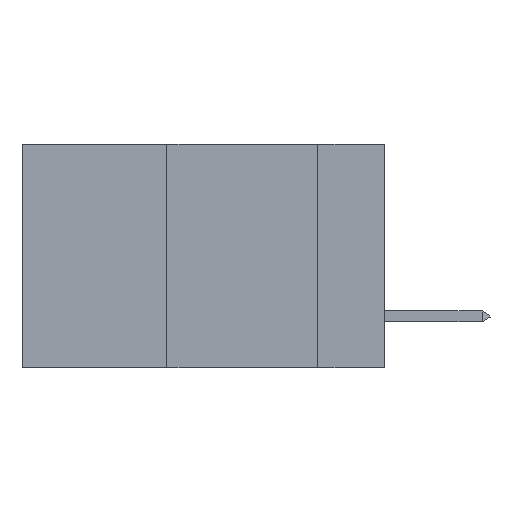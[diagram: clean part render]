
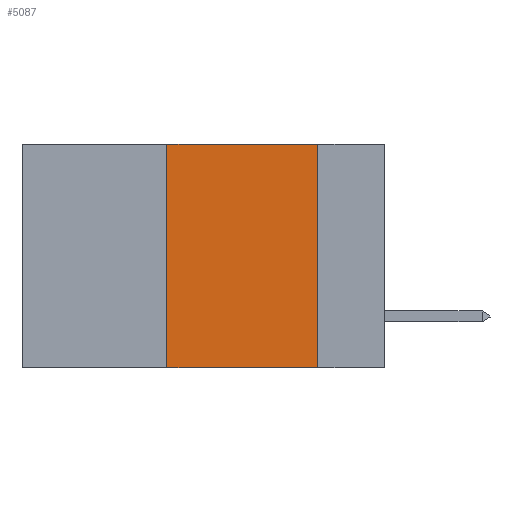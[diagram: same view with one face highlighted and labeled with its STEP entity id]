
A CAD part, left-side view. The second image highlights one B-rep face of the part: STEP entity #5087.
In plain terms, the highlighted planar face has unit normal (-1, 0, 0).
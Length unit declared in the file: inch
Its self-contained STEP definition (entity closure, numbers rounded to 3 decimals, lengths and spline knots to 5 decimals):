
#1336 = ORIENTED_EDGE ( 'NONE', *, *, #5442, .F. ) ;
#1429 = CARTESIAN_POINT ( 'NONE',  ( 0., 0.6, -0.37 ) ) ;
#1559 = LINE ( 'NONE', #3818, #13068 ) ;
#1743 = DIRECTION ( 'NONE',  ( 0., 0., 1. ) ) ;
#3305 = DIRECTION ( 'NONE',  ( 0., -1., 0. ) ) ;
#3705 = FACE_OUTER_BOUND ( 'NONE', #15469, .T. ) ;
#3818 = CARTESIAN_POINT ( 'NONE',  ( 0., 0.11, 0. ) ) ;
#4526 = CARTESIAN_POINT ( 'NONE',  ( 0., 0.6, 0. ) ) ;
#4666 = LINE ( 'NONE', #4526, #16384 ) ;
#4720 = VERTEX_POINT ( 'NONE', #7109 ) ;
#4814 = CARTESIAN_POINT ( 'NONE',  ( 0., 0.6, 0. ) ) ;
#5087 = ADVANCED_FACE ( 'NONE', ( #3705 ), #9902, .F. ) ;
#5442 = EDGE_CURVE ( 'NONE', #5704, #4720, #1559, .T. ) ;
#5704 = VERTEX_POINT ( 'NONE', #6829 ) ;
#6124 = DIRECTION ( 'NONE',  ( 1., 0., 0. ) ) ;
#6217 = CARTESIAN_POINT ( 'NONE',  ( 0., 0.36, 0. ) ) ;
#6248 = EDGE_CURVE ( 'NONE', #13581, #12804, #13221, .T. ) ;
#6829 = CARTESIAN_POINT ( 'NONE',  ( 0., 0.11, 0. ) ) ;
#6848 = ORIENTED_EDGE ( 'NONE', *, *, #14218, .F. ) ;
#7109 = CARTESIAN_POINT ( 'NONE',  ( 0., 0.11, -0.37 ) ) ;
#7263 = VECTOR ( 'NONE', #1743, 39.37008 ) ;
#7389 = EDGE_CURVE ( 'NONE', #13581, #4720, #12853, .T. ) ;
#8726 = ORIENTED_EDGE ( 'NONE', *, *, #6248, .F. ) ;
#8911 = ORIENTED_EDGE ( 'NONE', *, *, #7389, .T. ) ;
#9166 = DIRECTION ( 'NONE',  ( 0., -1., 0. ) ) ;
#9665 = VECTOR ( 'NONE', #9166, 39.37008 ) ;
#9902 = PLANE ( 'NONE',  #15212 ) ;
#12204 = CARTESIAN_POINT ( 'NONE',  ( 0., 0.36, -0.37 ) ) ;
#12804 = VERTEX_POINT ( 'NONE', #6217 ) ;
#12853 = LINE ( 'NONE', #1429, #9665 ) ;
#13068 = VECTOR ( 'NONE', #16360, 39.37008 ) ;
#13221 = LINE ( 'NONE', #15648, #7263 ) ;
#13581 = VERTEX_POINT ( 'NONE', #12204 ) ;
#14218 = EDGE_CURVE ( 'NONE', #12804, #5704, #4666, .T. ) ;
#14969 = DIRECTION ( 'NONE',  ( 0., 0., -1. ) ) ;
#15212 = AXIS2_PLACEMENT_3D ( 'NONE', #4814, #6124, #14969 ) ;
#15469 = EDGE_LOOP ( 'NONE', ( #1336, #6848, #8726, #8911 ) ) ;
#15648 = CARTESIAN_POINT ( 'NONE',  ( 0., 0.36, 0. ) ) ;
#16360 = DIRECTION ( 'NONE',  ( 0., 0., -1. ) ) ;
#16384 = VECTOR ( 'NONE', #3305, 39.37008 ) ;
